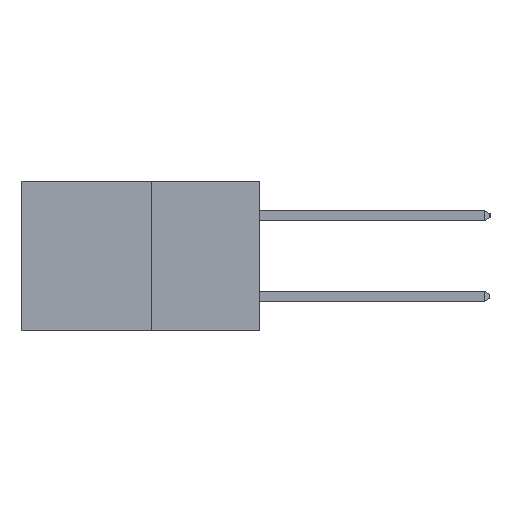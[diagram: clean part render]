
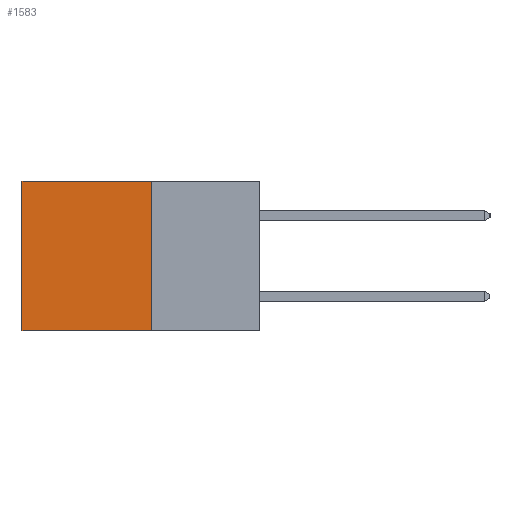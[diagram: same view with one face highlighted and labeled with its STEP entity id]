
A CAD part, left-side view. The second image highlights one B-rep face of the part: STEP entity #1583.
In plain terms, the highlighted planar face has unit normal (-1, 0, 0).
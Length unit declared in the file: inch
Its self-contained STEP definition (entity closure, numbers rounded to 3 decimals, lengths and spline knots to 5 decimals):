
#579 = DIRECTION ( 'NONE',  ( 0., 1., 0. ) ) ;
#714 = FACE_OUTER_BOUND ( 'NONE', #7195, .T. ) ;
#731 = DIRECTION ( 'NONE',  ( 0., 0., -1. ) ) ;
#744 = ORIENTED_EDGE ( 'NONE', *, *, #1307, .T. ) ;
#849 = CARTESIAN_POINT ( 'NONE',  ( 0.277, 0.27, 0. ) ) ;
#1143 = CARTESIAN_POINT ( 'NONE',  ( 0.277, 0.59, -0.37 ) ) ;
#1153 = CARTESIAN_POINT ( 'NONE',  ( 0.277, 0.27, -0.37 ) ) ;
#1307 = EDGE_CURVE ( 'NONE', #4426, #7439, #5760, .T. ) ;
#1569 = VECTOR ( 'NONE', #579, 39.37008 ) ;
#1583 = ADVANCED_FACE ( 'NONE', ( #714 ), #3042, .F. ) ;
#1673 = CARTESIAN_POINT ( 'NONE',  ( 0.277, 0.59, -0.37 ) ) ;
#2100 = ORIENTED_EDGE ( 'NONE', *, *, #5822, .T. ) ;
#2449 = ORIENTED_EDGE ( 'NONE', *, *, #3234, .F. ) ;
#2496 = ORIENTED_EDGE ( 'NONE', *, *, #4185, .F. ) ;
#2500 = LINE ( 'NONE', #6972, #3854 ) ;
#3042 = PLANE ( 'NONE',  #7908 ) ;
#3107 = VERTEX_POINT ( 'NONE', #849 ) ;
#3234 = EDGE_CURVE ( 'NONE', #5998, #7439, #2500, .T. ) ;
#3854 = VECTOR ( 'NONE', #5899, 39.37008 ) ;
#4077 = VECTOR ( 'NONE', #7101, 39.37008 ) ;
#4185 = EDGE_CURVE ( 'NONE', #3107, #5998, #4824, .T. ) ;
#4426 = VERTEX_POINT ( 'NONE', #6755 ) ;
#4824 = LINE ( 'NONE', #5944, #7836 ) ;
#4961 = DIRECTION ( 'NONE',  ( 1., 0., 0. ) ) ;
#5003 = LINE ( 'NONE', #7663, #1569 ) ;
#5760 = LINE ( 'NONE', #1143, #4077 ) ;
#5822 = EDGE_CURVE ( 'NONE', #3107, #4426, #5003, .T. ) ;
#5899 = DIRECTION ( 'NONE',  ( 0., 1., 0. ) ) ;
#5944 = CARTESIAN_POINT ( 'NONE',  ( 0.277, 0.27, -0.37 ) ) ;
#5998 = VERTEX_POINT ( 'NONE', #7232 ) ;
#6755 = CARTESIAN_POINT ( 'NONE',  ( 0.277, 0.59, 0. ) ) ;
#6972 = CARTESIAN_POINT ( 'NONE',  ( 0.277, 0.27, -0.37 ) ) ;
#6988 = DIRECTION ( 'NONE',  ( 0., 0., -1. ) ) ;
#7101 = DIRECTION ( 'NONE',  ( 0., 0., -1. ) ) ;
#7195 = EDGE_LOOP ( 'NONE', ( #744, #2449, #2496, #2100 ) ) ;
#7232 = CARTESIAN_POINT ( 'NONE',  ( 0.277, 0.27, -0.37 ) ) ;
#7439 = VERTEX_POINT ( 'NONE', #1673 ) ;
#7663 = CARTESIAN_POINT ( 'NONE',  ( 0.277, 0.27, 0. ) ) ;
#7836 = VECTOR ( 'NONE', #731, 39.37008 ) ;
#7908 = AXIS2_PLACEMENT_3D ( 'NONE', #1153, #4961, #6988 ) ;
